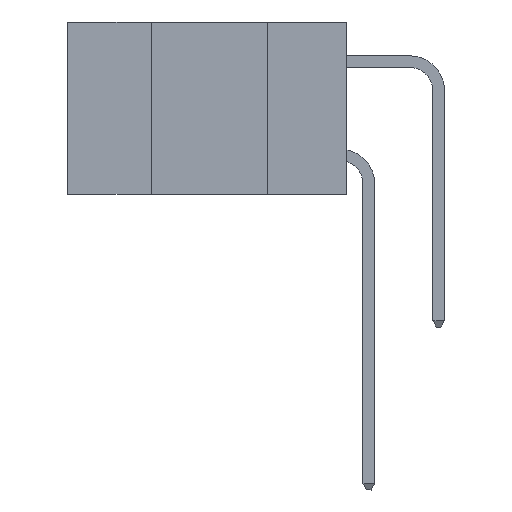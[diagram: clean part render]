
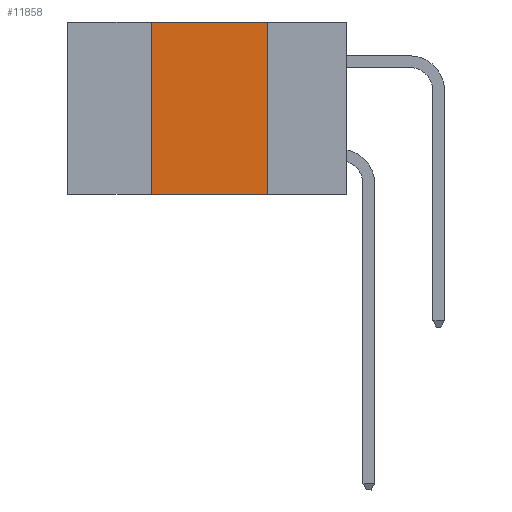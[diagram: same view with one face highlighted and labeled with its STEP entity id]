
A CAD part, left-side view. The second image highlights one B-rep face of the part: STEP entity #11858.
In plain terms, the highlighted planar face has unit normal (-1, 0, 0).
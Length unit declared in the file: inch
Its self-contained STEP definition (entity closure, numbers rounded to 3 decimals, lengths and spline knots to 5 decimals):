
#210 = EDGE_LOOP ( 'NONE', ( #1975, #8630, #10778, #6802 ) ) ;
#1489 = LINE ( 'NONE', #4388, #3281 ) ;
#1975 = ORIENTED_EDGE ( 'NONE', *, *, #4844, .F. ) ;
#2067 = EDGE_CURVE ( 'NONE', #5177, #10034, #1489, .T. ) ;
#2234 = CARTESIAN_POINT ( 'NONE',  ( 0., 0.6, 0. ) ) ;
#2269 = EDGE_CURVE ( 'NONE', #10034, #3246, #8792, .T. ) ;
#2361 = LINE ( 'NONE', #6084, #10169 ) ;
#2603 = VECTOR ( 'NONE', #11684, 39.37008 ) ;
#2662 = CARTESIAN_POINT ( 'NONE',  ( 0., 0.42, 0. ) ) ;
#3234 = DIRECTION ( 'NONE',  ( 0., 0., -1. ) ) ;
#3246 = VERTEX_POINT ( 'NONE', #6533 ) ;
#3281 = VECTOR ( 'NONE', #8421, 39.37008 ) ;
#4388 = CARTESIAN_POINT ( 'NONE',  ( 0., 0.42, 0. ) ) ;
#4718 = CARTESIAN_POINT ( 'NONE',  ( 0., 0.17, -0.37 ) ) ;
#4844 = EDGE_CURVE ( 'NONE', #3246, #7510, #2361, .T. ) ;
#5177 = VERTEX_POINT ( 'NONE', #5944 ) ;
#5286 = DIRECTION ( 'NONE',  ( 0., -1., 0. ) ) ;
#5944 = CARTESIAN_POINT ( 'NONE',  ( 0., 0.42, -0.37 ) ) ;
#6084 = CARTESIAN_POINT ( 'NONE',  ( 0., 0.17, 0. ) ) ;
#6239 = LINE ( 'NONE', #10066, #10635 ) ;
#6533 = CARTESIAN_POINT ( 'NONE',  ( 0., 0.17, 0. ) ) ;
#6675 = AXIS2_PLACEMENT_3D ( 'NONE', #8758, #11648, #8817 ) ;
#6802 = ORIENTED_EDGE ( 'NONE', *, *, #7458, .T. ) ;
#7458 = EDGE_CURVE ( 'NONE', #5177, #7510, #6239, .T. ) ;
#7510 = VERTEX_POINT ( 'NONE', #4718 ) ;
#8421 = DIRECTION ( 'NONE',  ( 0., 0., 1. ) ) ;
#8460 = FACE_OUTER_BOUND ( 'NONE', #210, .T. ) ;
#8630 = ORIENTED_EDGE ( 'NONE', *, *, #2269, .F. ) ;
#8758 = CARTESIAN_POINT ( 'NONE',  ( 0., 0.6, 0. ) ) ;
#8792 = LINE ( 'NONE', #2234, #2603 ) ;
#8817 = DIRECTION ( 'NONE',  ( 0., 0., -1. ) ) ;
#9760 = PLANE ( 'NONE',  #6675 ) ;
#10034 = VERTEX_POINT ( 'NONE', #2662 ) ;
#10066 = CARTESIAN_POINT ( 'NONE',  ( 0., 0.6, -0.37 ) ) ;
#10169 = VECTOR ( 'NONE', #3234, 39.37008 ) ;
#10635 = VECTOR ( 'NONE', #5286, 39.37008 ) ;
#10778 = ORIENTED_EDGE ( 'NONE', *, *, #2067, .F. ) ;
#11648 = DIRECTION ( 'NONE',  ( 1., 0., 0. ) ) ;
#11684 = DIRECTION ( 'NONE',  ( 0., -1., 0. ) ) ;
#11858 = ADVANCED_FACE ( 'NONE', ( #8460 ), #9760, .F. ) ;
